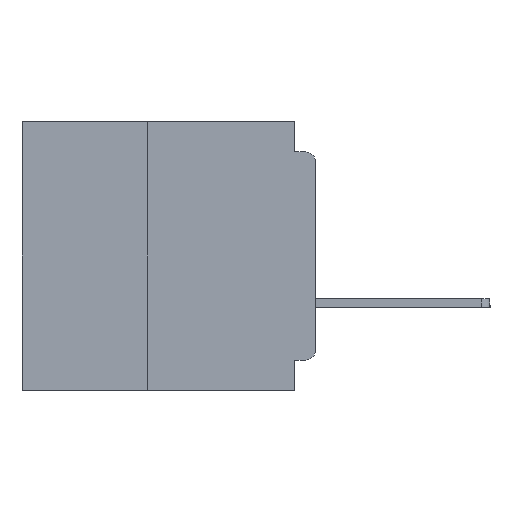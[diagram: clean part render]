
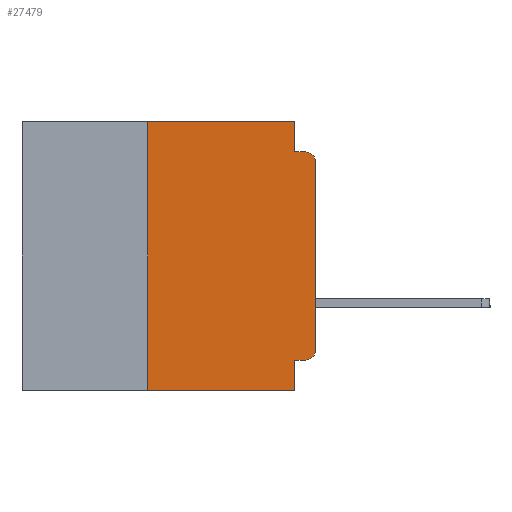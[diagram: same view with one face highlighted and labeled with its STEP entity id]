
A CAD part, left-side view. The second image highlights one B-rep face of the part: STEP entity #27479.
In plain terms, the highlighted planar face has unit normal (-1, 0, 0).
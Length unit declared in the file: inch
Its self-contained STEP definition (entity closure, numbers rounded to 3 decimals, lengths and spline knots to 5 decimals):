
#149 = CARTESIAN_POINT ( 'NONE',  ( 0., 0., -0.355 ) ) ;
#459 = LINE ( 'NONE', #29138, #66585 ) ;
#2164 = ORIENTED_EDGE ( 'NONE', *, *, #37793, .F. ) ;
#2410 = CARTESIAN_POINT ( 'NONE',  ( 0., 0., 0. ) ) ;
#2794 = DIRECTION ( 'NONE',  ( -1., 0., 0. ) ) ;
#2941 = CARTESIAN_POINT ( 'NONE',  ( 0., 0.031, -0.4 ) ) ;
#3157 = DIRECTION ( 'NONE',  ( 0., -1., 0. ) ) ;
#3976 = ORIENTED_EDGE ( 'NONE', *, *, #64623, .F. ) ;
#4162 = EDGE_CURVE ( 'NONE', #45603, #7846, #459, .T. ) ;
#4165 = DIRECTION ( 'NONE',  ( -1., 0., 0. ) ) ;
#4658 = EDGE_CURVE ( 'NONE', #42990, #13434, #35472, .T. ) ;
#5421 = DIRECTION ( 'NONE',  ( 0., 1., 0. ) ) ;
#6001 = VERTEX_POINT ( 'NONE', #29577 ) ;
#6050 = VECTOR ( 'NONE', #24492, 39.37008 ) ;
#6775 = DIRECTION ( 'NONE',  ( 0., 0., 1. ) ) ;
#7655 = DIRECTION ( 'NONE',  ( 0., 0., 1. ) ) ;
#7846 = VERTEX_POINT ( 'NONE', #28965 ) ;
#8093 = ORIENTED_EDGE ( 'NONE', *, *, #10577, .F. ) ;
#10297 = CARTESIAN_POINT ( 'NONE',  ( 0., 0.031, -0.045 ) ) ;
#10577 = EDGE_CURVE ( 'NONE', #14061, #24726, #18317, .T. ) ;
#13434 = VERTEX_POINT ( 'NONE', #20876 ) ;
#13911 = VECTOR ( 'NONE', #60805, 39.37008 ) ;
#14061 = VERTEX_POINT ( 'NONE', #10297 ) ;
#14318 = LINE ( 'NONE', #149, #26488 ) ;
#14387 = VECTOR ( 'NONE', #6775, 39.37008 ) ;
#14891 = DIRECTION ( 'NONE',  ( 0., 0., -1. ) ) ;
#16701 = LINE ( 'NONE', #54231, #41135 ) ;
#17836 = EDGE_CURVE ( 'NONE', #6001, #50386, #58692, .T. ) ;
#18317 = LINE ( 'NONE', #50569, #6050 ) ;
#19880 = CARTESIAN_POINT ( 'NONE',  ( 0., 0., -0.34 ) ) ;
#20766 = ORIENTED_EDGE ( 'NONE', *, *, #56180, .T. ) ;
#20876 = CARTESIAN_POINT ( 'NONE',  ( 0., 0., -0.06 ) ) ;
#22350 = AXIS2_PLACEMENT_3D ( 'NONE', #34033, #2794, #39283 ) ;
#23147 = CARTESIAN_POINT ( 'NONE',  ( 0., 0.015, -0.045 ) ) ;
#24492 = DIRECTION ( 'NONE',  ( 0., -1., 0. ) ) ;
#24726 = VERTEX_POINT ( 'NONE', #23147 ) ;
#26158 = ORIENTED_EDGE ( 'NONE', *, *, #4162, .F. ) ;
#26488 = VECTOR ( 'NONE', #5421, 39.37008 ) ;
#26563 = EDGE_CURVE ( 'NONE', #49487, #45603, #43742, .T. ) ;
#27479 = ADVANCED_FACE ( 'NONE', ( #55441 ), #40850, .F. ) ;
#27521 = ORIENTED_EDGE ( 'NONE', *, *, #26563, .F. ) ;
#28965 = CARTESIAN_POINT ( 'NONE',  ( 0., 0.031, 0. ) ) ;
#29138 = CARTESIAN_POINT ( 'NONE',  ( 0., 0.437, 0. ) ) ;
#29453 = CARTESIAN_POINT ( 'NONE',  ( 0., 0.437, -0.4 ) ) ;
#29577 = CARTESIAN_POINT ( 'NONE',  ( 0., 0.031, -0.355 ) ) ;
#30737 = AXIS2_PLACEMENT_3D ( 'NONE', #35391, #4165, #40648 ) ;
#32436 = EDGE_CURVE ( 'NONE', #35737, #42990, #34257, .T. ) ;
#34033 = CARTESIAN_POINT ( 'NONE',  ( 0., 0.015, -0.06 ) ) ;
#34112 = VECTOR ( 'NONE', #34179, 39.37008 ) ;
#34179 = DIRECTION ( 'NONE',  ( 0., 0., -1. ) ) ;
#34257 = CIRCLE ( 'NONE', #30737, 0.015 ) ;
#34561 = CARTESIAN_POINT ( 'NONE',  ( 0., 0.031, -0.4 ) ) ;
#35391 = CARTESIAN_POINT ( 'NONE',  ( 0., 0.015, -0.34 ) ) ;
#35472 = LINE ( 'NONE', #2410, #47811 ) ;
#35737 = VERTEX_POINT ( 'NONE', #62535 ) ;
#37793 = EDGE_CURVE ( 'NONE', #35737, #6001, #14318, .T. ) ;
#38593 = DIRECTION ( 'NONE',  ( 0., 0., -1. ) ) ;
#39283 = DIRECTION ( 'NONE',  ( 0., 0., -1. ) ) ;
#39957 = LINE ( 'NONE', #29453, #13911 ) ;
#40648 = DIRECTION ( 'NONE',  ( 0., 0., -1. ) ) ;
#40696 = CIRCLE ( 'NONE', #22350, 0.015 ) ;
#40850 = PLANE ( 'NONE',  #41434 ) ;
#41135 = VECTOR ( 'NONE', #38593, 39.37008 ) ;
#41434 = AXIS2_PLACEMENT_3D ( 'NONE', #56488, #46149, #14891 ) ;
#42990 = VERTEX_POINT ( 'NONE', #19880 ) ;
#43742 = LINE ( 'NONE', #48567, #14387 ) ;
#44169 = ORIENTED_EDGE ( 'NONE', *, *, #50910, .T. ) ;
#45603 = VERTEX_POINT ( 'NONE', #46211 ) ;
#46149 = DIRECTION ( 'NONE',  ( 1., 0., 0. ) ) ;
#46211 = CARTESIAN_POINT ( 'NONE',  ( 0., 0.25, 0. ) ) ;
#46509 = EDGE_LOOP ( 'NONE', ( #60577, #44169, #8093, #3976, #26158, #27521, #20766, #56295, #2164, #54144 ) ) ;
#47051 = CARTESIAN_POINT ( 'NONE',  ( 0., 0.25, -0.4 ) ) ;
#47811 = VECTOR ( 'NONE', #7655, 39.37008 ) ;
#48567 = CARTESIAN_POINT ( 'NONE',  ( 0., 0.25, -0.4 ) ) ;
#49487 = VERTEX_POINT ( 'NONE', #47051 ) ;
#50386 = VERTEX_POINT ( 'NONE', #34561 ) ;
#50569 = CARTESIAN_POINT ( 'NONE',  ( 0., 0., -0.045 ) ) ;
#50910 = EDGE_CURVE ( 'NONE', #13434, #24726, #40696, .T. ) ;
#54144 = ORIENTED_EDGE ( 'NONE', *, *, #32436, .T. ) ;
#54231 = CARTESIAN_POINT ( 'NONE',  ( 0., 0.031, 0. ) ) ;
#55441 = FACE_OUTER_BOUND ( 'NONE', #46509, .T. ) ;
#56180 = EDGE_CURVE ( 'NONE', #49487, #50386, #39957, .T. ) ;
#56295 = ORIENTED_EDGE ( 'NONE', *, *, #17836, .F. ) ;
#56488 = CARTESIAN_POINT ( 'NONE',  ( 0., 0.437, 0. ) ) ;
#58692 = LINE ( 'NONE', #2941, #34112 ) ;
#60577 = ORIENTED_EDGE ( 'NONE', *, *, #4658, .T. ) ;
#60805 = DIRECTION ( 'NONE',  ( 0., -1., 0. ) ) ;
#62535 = CARTESIAN_POINT ( 'NONE',  ( 0., 0.015, -0.355 ) ) ;
#64623 = EDGE_CURVE ( 'NONE', #7846, #14061, #16701, .T. ) ;
#66585 = VECTOR ( 'NONE', #3157, 39.37008 ) ;
